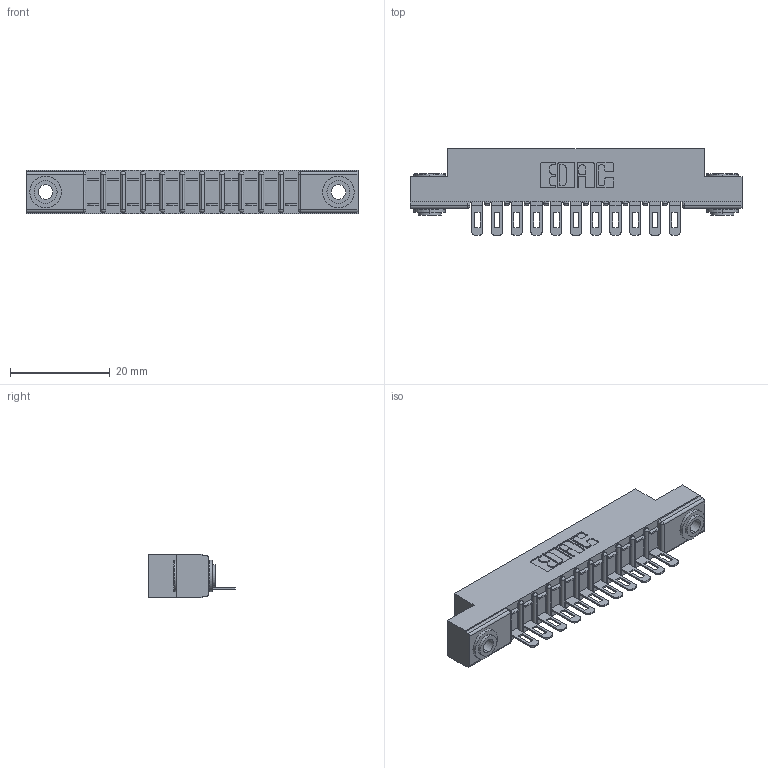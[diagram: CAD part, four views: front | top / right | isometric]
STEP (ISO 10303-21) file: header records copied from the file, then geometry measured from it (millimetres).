
FILE_DESCRIPTION (( 'STEP AP203' ), '1' );
FILE_NAME ('307-011-401-103.STEP', '2020-09-25T09:56:14', ( '' ), ( '' ), 'SwSTEP 2.0', 'SolidWorks 2020', '' );
FILE_SCHEMA (( 'CONFIG_CONTROL_DESIGN' ));
Length unit declared in the file: inch
Products named in the file (4): 307 Part_.156 Dia Mounting Holes; 307-290-002_501; 307-011-401-103; 345-250-002_345-250-002-102
Assembly tree (14 placements, depth 2):
  307-011-401-103
    307 Part_.156 Dia Mounting Holes
    307-290-002_501  x11
    345-250-002_345-250-002-102  x2
Bounding box: 66.6 x 17.42 x 8.71 mm (x, y, z)
Volume: 4401.8 mm3; surface area: 7712.6 mm2
Topology: 14 solids, 14 shells, 1018 faces, 3053 edges, 1998 vertices
Faces by surface type: plane 578, cylinder 408, sphere 24, cone 8
Entity records: 15111 total; most frequent: CARTESIAN_POINT 2521, ORIENTED_EDGE 2502, DIRECTION 2483, EDGE_CURVE 1251, VECTOR 931, LINE 931, VERTEX_POINT 814, AXIS2_PLACEMENT_3D 776
